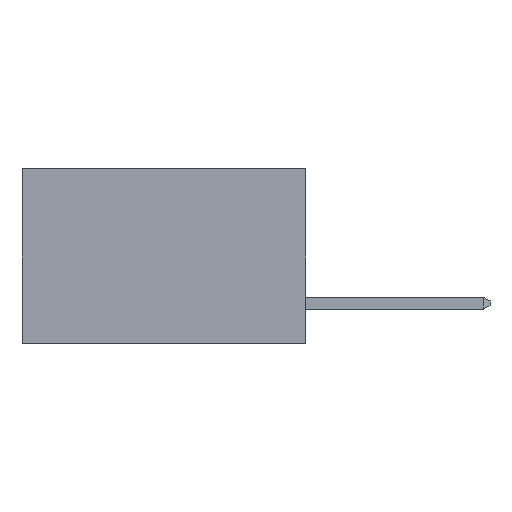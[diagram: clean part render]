
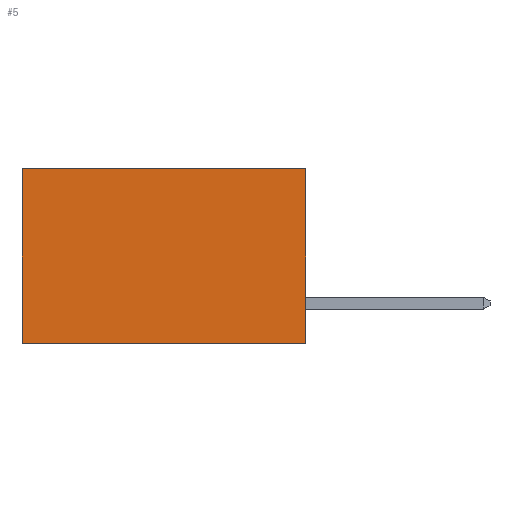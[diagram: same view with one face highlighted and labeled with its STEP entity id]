
A CAD part, left-side view. The second image highlights one B-rep face of the part: STEP entity #5.
In plain terms, the highlighted planar face has unit normal (-1, 0, 0).
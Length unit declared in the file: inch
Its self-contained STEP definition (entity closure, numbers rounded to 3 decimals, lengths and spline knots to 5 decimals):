
#5 = ADVANCED_FACE ( 'NONE', ( #2009 ), #18347, .F. ) ;
#1367 = EDGE_LOOP ( 'NONE', ( #5588, #11814, #11925, #3706 ) ) ;
#1885 = CARTESIAN_POINT ( 'NONE',  ( 0.2615, 0., 0. ) ) ;
#2009 = FACE_OUTER_BOUND ( 'NONE', #1367, .T. ) ;
#3388 = DIRECTION ( 'NONE',  ( 0., 1., 0. ) ) ;
#3506 = VERTEX_POINT ( 'NONE', #5146 ) ;
#3706 = ORIENTED_EDGE ( 'NONE', *, *, #10443, .T. ) ;
#5146 = CARTESIAN_POINT ( 'NONE',  ( 0.2615, 0., -0.37 ) ) ;
#5588 = ORIENTED_EDGE ( 'NONE', *, *, #7144, .T. ) ;
#7144 = EDGE_CURVE ( 'NONE', #7629, #16834, #14494, .T. ) ;
#7629 = VERTEX_POINT ( 'NONE', #7996 ) ;
#7911 = DIRECTION ( 'NONE',  ( 0., 0., -1. ) ) ;
#7996 = CARTESIAN_POINT ( 'NONE',  ( 0.2615, 0.6, 0. ) ) ;
#8039 = VECTOR ( 'NONE', #12858, 39.37008 ) ;
#8794 = DIRECTION ( 'NONE',  ( 0., 0., -1. ) ) ;
#9422 = LINE ( 'NONE', #18836, #12442 ) ;
#10443 = EDGE_CURVE ( 'NONE', #18440, #7629, #16350, .T. ) ;
#11814 = ORIENTED_EDGE ( 'NONE', *, *, #18606, .F. ) ;
#11925 = ORIENTED_EDGE ( 'NONE', *, *, #13371, .F. ) ;
#12277 = DIRECTION ( 'NONE',  ( 1., 0., 0. ) ) ;
#12442 = VECTOR ( 'NONE', #8794, 39.37008 ) ;
#12493 = LINE ( 'NONE', #17118, #8039 ) ;
#12527 = VECTOR ( 'NONE', #3388, 39.37008 ) ;
#12858 = DIRECTION ( 'NONE',  ( 0., 1., 0. ) ) ;
#13174 = CARTESIAN_POINT ( 'NONE',  ( 0.2615, 0., -0.37 ) ) ;
#13371 = EDGE_CURVE ( 'NONE', #18440, #3506, #9422, .T. ) ;
#14031 = VECTOR ( 'NONE', #7911, 39.37008 ) ;
#14494 = LINE ( 'NONE', #17184, #14031 ) ;
#14696 = AXIS2_PLACEMENT_3D ( 'NONE', #13174, #12277, #17544 ) ;
#16350 = LINE ( 'NONE', #1885, #12527 ) ;
#16740 = CARTESIAN_POINT ( 'NONE',  ( 0.2615, 0., 0. ) ) ;
#16834 = VERTEX_POINT ( 'NONE', #18828 ) ;
#17118 = CARTESIAN_POINT ( 'NONE',  ( 0.2615, 0., -0.37 ) ) ;
#17184 = CARTESIAN_POINT ( 'NONE',  ( 0.2615, 0.6, -0.37 ) ) ;
#17544 = DIRECTION ( 'NONE',  ( 0., 0., -1. ) ) ;
#18347 = PLANE ( 'NONE',  #14696 ) ;
#18440 = VERTEX_POINT ( 'NONE', #16740 ) ;
#18606 = EDGE_CURVE ( 'NONE', #3506, #16834, #12493, .T. ) ;
#18828 = CARTESIAN_POINT ( 'NONE',  ( 0.2615, 0.6, -0.37 ) ) ;
#18836 = CARTESIAN_POINT ( 'NONE',  ( 0.2615, 0., -0.37 ) ) ;
